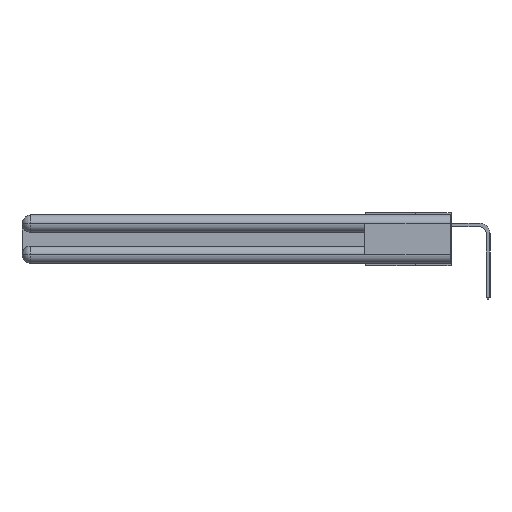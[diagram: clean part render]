
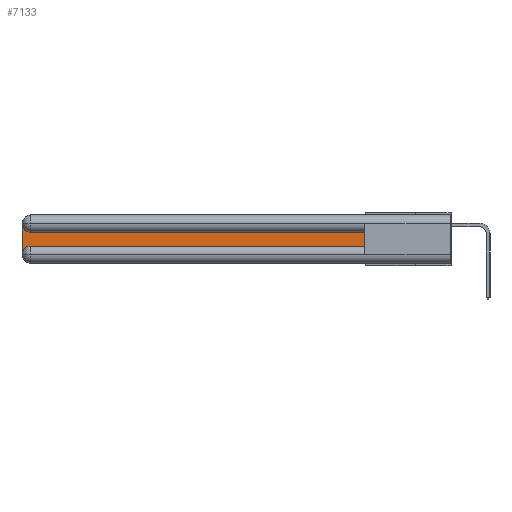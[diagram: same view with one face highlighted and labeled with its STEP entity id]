
A CAD part, left-side view. The second image highlights one B-rep face of the part: STEP entity #7133.
In plain terms, the highlighted planar face has unit normal (-1, 0, 0).
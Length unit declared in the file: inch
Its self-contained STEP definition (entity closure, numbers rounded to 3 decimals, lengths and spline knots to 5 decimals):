
#259 = CARTESIAN_POINT ( 'NONE',  ( 0.075, 2.94, -0.2775 ) ) ;
#744 = LINE ( 'NONE', #8395, #17360 ) ;
#752 = CIRCLE ( 'NONE', #13911, 0.06 ) ;
#1752 = LINE ( 'NONE', #22270, #11761 ) ;
#1780 = EDGE_CURVE ( 'NONE', #3314, #3997, #7950, .T. ) ;
#2666 = CIRCLE ( 'NONE', #20161, 0.06 ) ;
#3063 = ORIENTED_EDGE ( 'NONE', *, *, #16111, .T. ) ;
#3214 = VERTEX_POINT ( 'NONE', #21797 ) ;
#3314 = VERTEX_POINT ( 'NONE', #8054 ) ;
#3447 = CARTESIAN_POINT ( 'NONE',  ( 0.075, 0.6, -0.2175 ) ) ;
#3534 = EDGE_LOOP ( 'NONE', ( #3063, #25907, #12303, #8194, #5535, #24783 ) ) ;
#3994 = CARTESIAN_POINT ( 'NONE',  ( 0.075, 3., -0.2175 ) ) ;
#3997 = VERTEX_POINT ( 'NONE', #23389 ) ;
#4762 = CARTESIAN_POINT ( 'NONE',  ( 0.075, 0.6, -0.1225 ) ) ;
#4998 = DIRECTION ( 'NONE',  ( 0., 0., -1. ) ) ;
#5096 = VERTEX_POINT ( 'NONE', #4762 ) ;
#5535 = ORIENTED_EDGE ( 'NONE', *, *, #8806, .T. ) ;
#6234 = DIRECTION ( 'NONE',  ( 1., 0., 0. ) ) ;
#7133 = ADVANCED_FACE ( 'NONE', ( #15558 ), #17239, .F. ) ;
#7950 = LINE ( 'NONE', #3994, #12000 ) ;
#8054 = CARTESIAN_POINT ( 'NONE',  ( 0.075, 3., -0.0625 ) ) ;
#8194 = ORIENTED_EDGE ( 'NONE', *, *, #24112, .T. ) ;
#8376 = CARTESIAN_POINT ( 'NONE',  ( 0.075, 2.94, -0.0625 ) ) ;
#8395 = CARTESIAN_POINT ( 'NONE',  ( 0.075, 0.6, -0.2175 ) ) ;
#8806 = EDGE_CURVE ( 'NONE', #22104, #15947, #744, .T. ) ;
#10311 = DIRECTION ( 'NONE',  ( 1., 0., 0. ) ) ;
#10587 = DIRECTION ( 'NONE',  ( 0., -1., 0. ) ) ;
#11761 = VECTOR ( 'NONE', #24435, 39.37008 ) ;
#12000 = VECTOR ( 'NONE', #20019, 39.37008 ) ;
#12303 = ORIENTED_EDGE ( 'NONE', *, *, #1780, .T. ) ;
#13019 = CARTESIAN_POINT ( 'NONE',  ( 0.075, 3., -0.1225 ) ) ;
#13024 = DIRECTION ( 'NONE',  ( 0., 0., 1. ) ) ;
#13911 = AXIS2_PLACEMENT_3D ( 'NONE', #8376, #10311, #20607 ) ;
#15558 = FACE_OUTER_BOUND ( 'NONE', #3534, .T. ) ;
#15947 = VERTEX_POINT ( 'NONE', #3447 ) ;
#16111 = EDGE_CURVE ( 'NONE', #5096, #3214, #1752, .T. ) ;
#16301 = DIRECTION ( 'NONE',  ( 0., 0., -1. ) ) ;
#17239 = PLANE ( 'NONE',  #17382 ) ;
#17360 = VECTOR ( 'NONE', #10587, 39.37008 ) ;
#17382 = AXIS2_PLACEMENT_3D ( 'NONE', #13019, #23114, #4998 ) ;
#17838 = EDGE_CURVE ( 'NONE', #15947, #5096, #23454, .T. ) ;
#18509 = CARTESIAN_POINT ( 'NONE',  ( 0.075, 2.94, -0.2175 ) ) ;
#19353 = CARTESIAN_POINT ( 'NONE',  ( 0.075, 0.6, -0.2175 ) ) ;
#20019 = DIRECTION ( 'NONE',  ( 0., 0., -1. ) ) ;
#20161 = AXIS2_PLACEMENT_3D ( 'NONE', #259, #6234, #16301 ) ;
#20607 = DIRECTION ( 'NONE',  ( 0., 0., -1. ) ) ;
#21797 = CARTESIAN_POINT ( 'NONE',  ( 0.075, 2.94, -0.1225 ) ) ;
#22104 = VERTEX_POINT ( 'NONE', #18509 ) ;
#22270 = CARTESIAN_POINT ( 'NONE',  ( 0.075, 0.6, -0.1225 ) ) ;
#23114 = DIRECTION ( 'NONE',  ( 1., 0., 0. ) ) ;
#23389 = CARTESIAN_POINT ( 'NONE',  ( 0.075, 3., -0.2775 ) ) ;
#23454 = LINE ( 'NONE', #19353, #24080 ) ;
#23596 = EDGE_CURVE ( 'NONE', #3214, #3314, #752, .T. ) ;
#24080 = VECTOR ( 'NONE', #13024, 39.37008 ) ;
#24112 = EDGE_CURVE ( 'NONE', #3997, #22104, #2666, .T. ) ;
#24435 = DIRECTION ( 'NONE',  ( 0., 1., 0. ) ) ;
#24783 = ORIENTED_EDGE ( 'NONE', *, *, #17838, .T. ) ;
#25907 = ORIENTED_EDGE ( 'NONE', *, *, #23596, .T. ) ;
